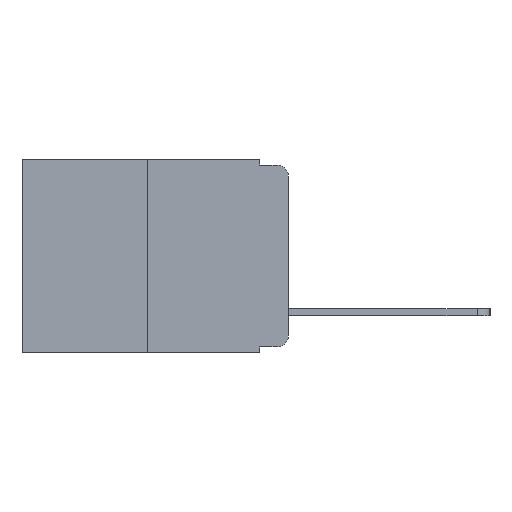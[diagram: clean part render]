
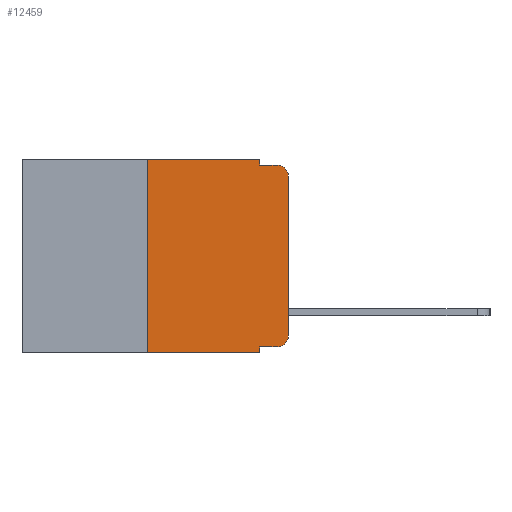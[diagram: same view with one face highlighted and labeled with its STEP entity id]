
A CAD part, left-side view. The second image highlights one B-rep face of the part: STEP entity #12459.
In plain terms, the highlighted planar face has unit normal (-1, 0, 0).
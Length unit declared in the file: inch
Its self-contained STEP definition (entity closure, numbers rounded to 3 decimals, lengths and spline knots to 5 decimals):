
#637 = EDGE_CURVE ( 'NONE', #18363, #13156, #19051, .T. ) ;
#859 = VECTOR ( 'NONE', #1176, 39.37008 ) ;
#952 = DIRECTION ( 'NONE',  ( 0., 0., -1. ) ) ;
#1176 = DIRECTION ( 'NONE',  ( 0., -1., 0. ) ) ;
#2021 = CARTESIAN_POINT ( 'NONE',  ( 0., 0.25, 0. ) ) ;
#2293 = CARTESIAN_POINT ( 'NONE',  ( 0., 0., 0. ) ) ;
#2310 = ORIENTED_EDGE ( 'NONE', *, *, #5279, .F. ) ;
#2599 = VECTOR ( 'NONE', #9910, 39.37008 ) ;
#3512 = AXIS2_PLACEMENT_3D ( 'NONE', #18866, #14315, #4745 ) ;
#4090 = VERTEX_POINT ( 'NONE', #13903 ) ;
#4210 = ORIENTED_EDGE ( 'NONE', *, *, #20344, .T. ) ;
#4292 = FACE_OUTER_BOUND ( 'NONE', #17495, .T. ) ;
#4421 = CARTESIAN_POINT ( 'NONE',  ( 0., 0.02, -0.03 ) ) ;
#4606 = DIRECTION ( 'NONE',  ( -1., 0., 0. ) ) ;
#4643 = CARTESIAN_POINT ( 'NONE',  ( 0., 0.051, -0.343 ) ) ;
#4730 = ORIENTED_EDGE ( 'NONE', *, *, #16275, .T. ) ;
#4745 = DIRECTION ( 'NONE',  ( 0., 0., -1. ) ) ;
#5095 = LINE ( 'NONE', #2293, #8410 ) ;
#5264 = VERTEX_POINT ( 'NONE', #13324 ) ;
#5279 = EDGE_CURVE ( 'NONE', #15102, #5525, #10375, .T. ) ;
#5525 = VERTEX_POINT ( 'NONE', #18673 ) ;
#5799 = CARTESIAN_POINT ( 'NONE',  ( 0., 0.473, -0.343 ) ) ;
#6005 = ORIENTED_EDGE ( 'NONE', *, *, #20735, .T. ) ;
#6069 = DIRECTION ( 'NONE',  ( 0., 0., -1. ) ) ;
#6685 = LINE ( 'NONE', #20671, #10440 ) ;
#7050 = DIRECTION ( 'NONE',  ( 0., 0., 1. ) ) ;
#7237 = ORIENTED_EDGE ( 'NONE', *, *, #10648, .T. ) ;
#7797 = CARTESIAN_POINT ( 'NONE',  ( 0., 0.051, -0.333 ) ) ;
#8052 = VERTEX_POINT ( 'NONE', #14178 ) ;
#8410 = VECTOR ( 'NONE', #15194, 39.37008 ) ;
#8545 = EDGE_CURVE ( 'NONE', #8052, #5264, #19042, .T. ) ;
#8629 = VERTEX_POINT ( 'NONE', #17296 ) ;
#8730 = VERTEX_POINT ( 'NONE', #11482 ) ;
#8753 = CIRCLE ( 'NONE', #12139, 0.02 ) ;
#9555 = PLANE ( 'NONE',  #3512 ) ;
#9602 = EDGE_CURVE ( 'NONE', #5264, #8629, #11283, .T. ) ;
#9910 = DIRECTION ( 'NONE',  ( 0., -1., 0. ) ) ;
#10375 = LINE ( 'NONE', #2021, #18138 ) ;
#10440 = VECTOR ( 'NONE', #14640, 39.37008 ) ;
#10594 = CIRCLE ( 'NONE', #14199, 0.02 ) ;
#10648 = EDGE_CURVE ( 'NONE', #12161, #8629, #8753, .T. ) ;
#11283 = LINE ( 'NONE', #20627, #2599 ) ;
#11332 = CARTESIAN_POINT ( 'NONE',  ( 0., 0.25, -0.343 ) ) ;
#11482 = CARTESIAN_POINT ( 'NONE',  ( 0., 0.02, -0.333 ) ) ;
#11737 = EDGE_CURVE ( 'NONE', #4090, #12161, #5095, .T. ) ;
#11925 = VECTOR ( 'NONE', #19867, 39.37008 ) ;
#12139 = AXIS2_PLACEMENT_3D ( 'NONE', #4421, #15561, #6069 ) ;
#12161 = VERTEX_POINT ( 'NONE', #19194 ) ;
#12459 = ADVANCED_FACE ( 'NONE', ( #4292 ), #9555, .F. ) ;
#13120 = CARTESIAN_POINT ( 'NONE',  ( 0., 0.051, 0. ) ) ;
#13156 = VERTEX_POINT ( 'NONE', #4643 ) ;
#13324 = CARTESIAN_POINT ( 'NONE',  ( 0., 0.051, -0.01 ) ) ;
#13902 = LINE ( 'NONE', #20280, #859 ) ;
#13903 = CARTESIAN_POINT ( 'NONE',  ( 0., 0., -0.313 ) ) ;
#14178 = CARTESIAN_POINT ( 'NONE',  ( 0., 0.051, 0. ) ) ;
#14194 = CARTESIAN_POINT ( 'NONE',  ( 0., 0.02, -0.313 ) ) ;
#14199 = AXIS2_PLACEMENT_3D ( 'NONE', #14194, #4606, #15731 ) ;
#14315 = DIRECTION ( 'NONE',  ( 1., 0., 0. ) ) ;
#14474 = ORIENTED_EDGE ( 'NONE', *, *, #637, .F. ) ;
#14640 = DIRECTION ( 'NONE',  ( 0., -1., 0. ) ) ;
#14699 = ORIENTED_EDGE ( 'NONE', *, *, #11737, .T. ) ;
#14994 = VECTOR ( 'NONE', #17646, 39.37008 ) ;
#15102 = VERTEX_POINT ( 'NONE', #11332 ) ;
#15194 = DIRECTION ( 'NONE',  ( 0., 0., 1. ) ) ;
#15411 = ORIENTED_EDGE ( 'NONE', *, *, #8545, .F. ) ;
#15561 = DIRECTION ( 'NONE',  ( -1., 0., 0. ) ) ;
#15582 = CARTESIAN_POINT ( 'NONE',  ( 0., 0.051, 0. ) ) ;
#15731 = DIRECTION ( 'NONE',  ( 0., 0., -1. ) ) ;
#16275 = EDGE_CURVE ( 'NONE', #8730, #4090, #10594, .T. ) ;
#16366 = ORIENTED_EDGE ( 'NONE', *, *, #20150, .F. ) ;
#17296 = CARTESIAN_POINT ( 'NONE',  ( 0., 0.02, -0.01 ) ) ;
#17495 = EDGE_LOOP ( 'NONE', ( #14699, #7237, #18999, #15411, #16366, #2310, #6005, #14474, #4210, #4730 ) ) ;
#17646 = DIRECTION ( 'NONE',  ( 0., 0., -1. ) ) ;
#18138 = VECTOR ( 'NONE', #7050, 39.37008 ) ;
#18363 = VERTEX_POINT ( 'NONE', #7797 ) ;
#18547 = VECTOR ( 'NONE', #952, 39.37008 ) ;
#18673 = CARTESIAN_POINT ( 'NONE',  ( 0., 0.25, 0. ) ) ;
#18866 = CARTESIAN_POINT ( 'NONE',  ( 0., 0.473, 0. ) ) ;
#18999 = ORIENTED_EDGE ( 'NONE', *, *, #9602, .F. ) ;
#19042 = LINE ( 'NONE', #15582, #18547 ) ;
#19051 = LINE ( 'NONE', #13120, #14994 ) ;
#19194 = CARTESIAN_POINT ( 'NONE',  ( 0., 0., -0.03 ) ) ;
#19867 = DIRECTION ( 'NONE',  ( 0., -1., 0. ) ) ;
#20095 = LINE ( 'NONE', #5799, #11925 ) ;
#20150 = EDGE_CURVE ( 'NONE', #5525, #8052, #13902, .T. ) ;
#20280 = CARTESIAN_POINT ( 'NONE',  ( 0., 0.473, 0. ) ) ;
#20344 = EDGE_CURVE ( 'NONE', #18363, #8730, #6685, .T. ) ;
#20627 = CARTESIAN_POINT ( 'NONE',  ( 0., 0.051, -0.01 ) ) ;
#20671 = CARTESIAN_POINT ( 'NONE',  ( 0., 0.051, -0.333 ) ) ;
#20735 = EDGE_CURVE ( 'NONE', #15102, #13156, #20095, .T. ) ;
